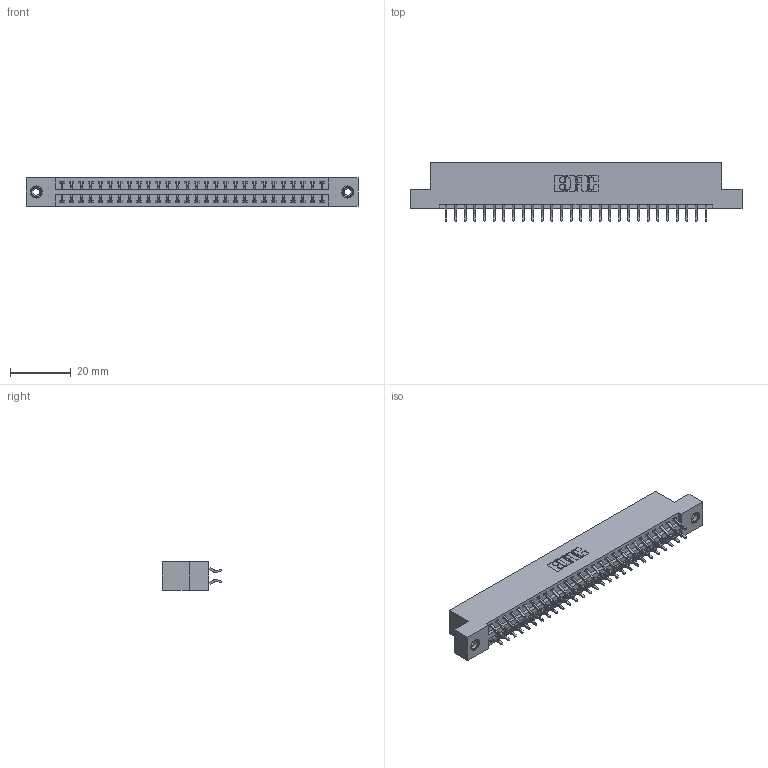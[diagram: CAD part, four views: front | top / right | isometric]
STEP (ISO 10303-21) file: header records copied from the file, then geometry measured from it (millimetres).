
FILE_DESCRIPTION (( 'STEP AP203' ), '1' );
FILE_NAME ('396-056-556-208.STEP', '2019-10-30T15:51:06', ( '' ), ( '' ), 'SwSTEP 2.0', 'SolidWorks 2016', '' );
FILE_SCHEMA (( 'CONFIG_CONTROL_DESIGN' ));
Length unit declared in the file: inch
Products named in the file (4): 346 Part_Flush Mounting Lugs - 0.156 Dia-TI; 345-292-001_556 Tail; 345-250-001_345-250-003-102; 396-056-556-208
Assembly tree (59 placements, depth 2):
  396-056-556-208
    346 Part_Flush Mounting Lugs - 0.156 Dia-TI
    345-292-001_556 Tail  x56
    345-250-001_345-250-003-102  x2
Bounding box: 109.47 x 19.57 x 9.4 mm (x, y, z)
Volume: 10557.6 mm3; surface area: 14260.1 mm2
Topology: 59 solids, 59 shells, 3430 faces, 10153 edges, 6686 vertices
Faces by surface type: plane 2292, cylinder 1122, cone 12, torus 4
Entity records: 21564 total; most frequent: CARTESIAN_POINT 3571, ORIENTED_EDGE 3486, DIRECTION 3213, EDGE_CURVE 1743, VECTOR 1471, LINE 1471, VERTEX_POINT 1156, AXIS2_PLACEMENT_3D 871
